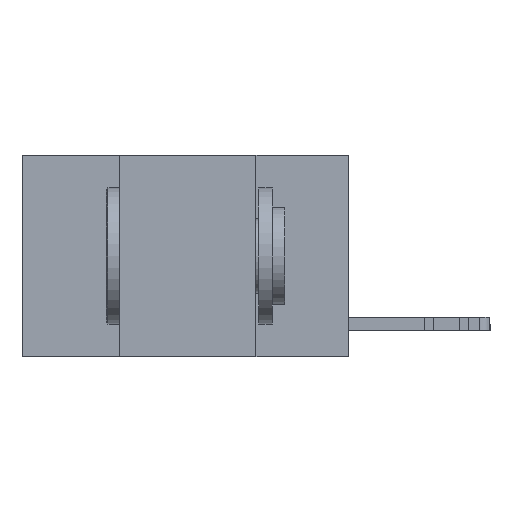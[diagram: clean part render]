
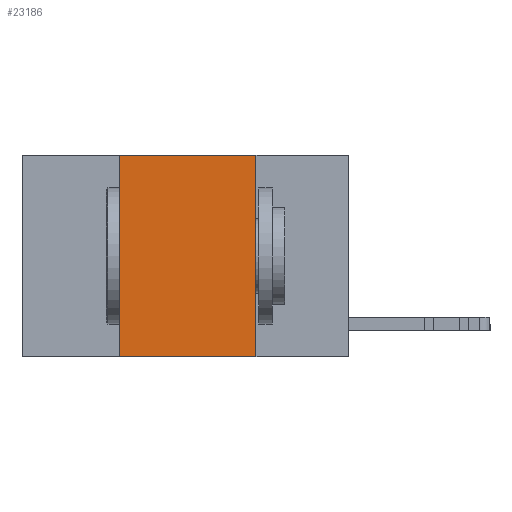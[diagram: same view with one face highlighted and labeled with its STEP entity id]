
A CAD part, left-side view. The second image highlights one B-rep face of the part: STEP entity #23186.
In plain terms, the highlighted planar face has unit normal (-1, 0, 0).
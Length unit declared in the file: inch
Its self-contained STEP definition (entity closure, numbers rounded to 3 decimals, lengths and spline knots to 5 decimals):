
#168 = DIRECTION ( 'NONE',  ( 0., -1., 0. ) ) ;
#961 = DIRECTION ( 'NONE',  ( 0., 0., -1. ) ) ;
#1254 = AXIS2_PLACEMENT_3D ( 'NONE', #18472, #16240, #27398 ) ;
#1666 = ORIENTED_EDGE ( 'NONE', *, *, #24658, .F. ) ;
#1789 = VERTEX_POINT ( 'NONE', #8269 ) ;
#2135 = FACE_OUTER_BOUND ( 'NONE', #20888, .T. ) ;
#3815 = DIRECTION ( 'NONE',  ( 0., 0., 1. ) ) ;
#4310 = EDGE_CURVE ( 'NONE', #21368, #1789, #16589, .T. ) ;
#4554 = CARTESIAN_POINT ( 'NONE',  ( 0., 0.6, -0.37 ) ) ;
#4878 = VECTOR ( 'NONE', #961, 39.37008 ) ;
#5773 = CARTESIAN_POINT ( 'NONE',  ( 0., 0.42, 0. ) ) ;
#7099 = LINE ( 'NONE', #4554, #11746 ) ;
#7747 = CARTESIAN_POINT ( 'NONE',  ( 0., 0.17, 0. ) ) ;
#8048 = CARTESIAN_POINT ( 'NONE',  ( 0., 0.42, -0.37 ) ) ;
#8269 = CARTESIAN_POINT ( 'NONE',  ( 0., 0.17, -0.37 ) ) ;
#9353 = PLANE ( 'NONE',  #1254 ) ;
#11746 = VECTOR ( 'NONE', #168, 39.37008 ) ;
#13410 = DIRECTION ( 'NONE',  ( 0., -1., 0. ) ) ;
#14137 = VECTOR ( 'NONE', #3815, 39.37008 ) ;
#14296 = ORIENTED_EDGE ( 'NONE', *, *, #17419, .T. ) ;
#14659 = ORIENTED_EDGE ( 'NONE', *, *, #21099, .F. ) ;
#15093 = LINE ( 'NONE', #5773, #14137 ) ;
#15234 = VECTOR ( 'NONE', #13410, 39.37008 ) ;
#16240 = DIRECTION ( 'NONE',  ( 1., 0., 0. ) ) ;
#16589 = LINE ( 'NONE', #7747, #4878 ) ;
#16688 = CARTESIAN_POINT ( 'NONE',  ( 0., 0.6, 0. ) ) ;
#17419 = EDGE_CURVE ( 'NONE', #21017, #1789, #7099, .T. ) ;
#18049 = ORIENTED_EDGE ( 'NONE', *, *, #4310, .F. ) ;
#18472 = CARTESIAN_POINT ( 'NONE',  ( 0., 0.6, 0. ) ) ;
#20888 = EDGE_LOOP ( 'NONE', ( #18049, #1666, #14659, #14296 ) ) ;
#21017 = VERTEX_POINT ( 'NONE', #8048 ) ;
#21099 = EDGE_CURVE ( 'NONE', #21017, #23267, #15093, .T. ) ;
#21368 = VERTEX_POINT ( 'NONE', #27690 ) ;
#23186 = ADVANCED_FACE ( 'NONE', ( #2135 ), #9353, .F. ) ;
#23267 = VERTEX_POINT ( 'NONE', #28572 ) ;
#24658 = EDGE_CURVE ( 'NONE', #23267, #21368, #28128, .T. ) ;
#27398 = DIRECTION ( 'NONE',  ( 0., 0., -1. ) ) ;
#27690 = CARTESIAN_POINT ( 'NONE',  ( 0., 0.17, 0. ) ) ;
#28128 = LINE ( 'NONE', #16688, #15234 ) ;
#28572 = CARTESIAN_POINT ( 'NONE',  ( 0., 0.42, 0. ) ) ;
